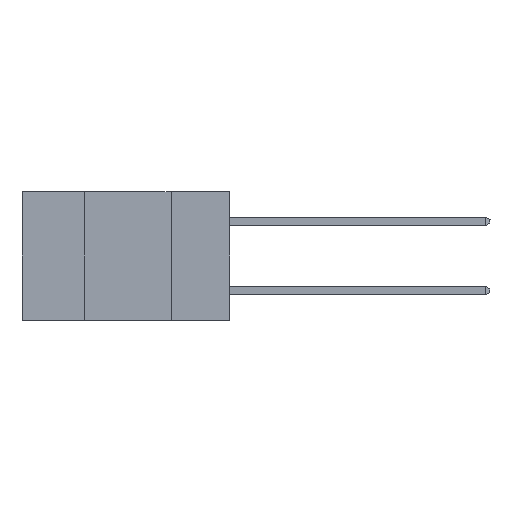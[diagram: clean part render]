
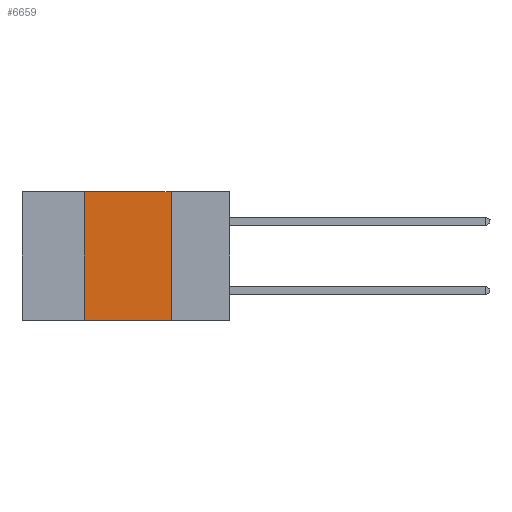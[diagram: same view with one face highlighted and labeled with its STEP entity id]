
A CAD part, left-side view. The second image highlights one B-rep face of the part: STEP entity #6659.
In plain terms, the highlighted planar face has unit normal (-1, 0, 0).
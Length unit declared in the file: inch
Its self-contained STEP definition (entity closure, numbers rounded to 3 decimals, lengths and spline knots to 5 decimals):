
#27 = DIRECTION ( 'NONE',  ( 0., 0., -1. ) ) ;
#76 = ORIENTED_EDGE ( 'NONE', *, *, #216, .T. ) ;
#216 = EDGE_CURVE ( 'NONE', #8223, #8405, #10692, .T. ) ;
#266 = CARTESIAN_POINT ( 'NONE',  ( 0., 0.17, 0. ) ) ;
#693 = EDGE_CURVE ( 'NONE', #8223, #9026, #9297, .T. ) ;
#1238 = DIRECTION ( 'NONE',  ( 1., 0., 0. ) ) ;
#1848 = VECTOR ( 'NONE', #7235, 39.37008 ) ;
#2009 = PLANE ( 'NONE',  #9515 ) ;
#2565 = EDGE_CURVE ( 'NONE', #7251, #8405, #10764, .T. ) ;
#2962 = DIRECTION ( 'NONE',  ( 0., -1., 0. ) ) ;
#3713 = VECTOR ( 'NONE', #4047, 39.37008 ) ;
#4047 = DIRECTION ( 'NONE',  ( 0., -1., 0. ) ) ;
#5865 = CARTESIAN_POINT ( 'NONE',  ( 0., 0.6, 0. ) ) ;
#6057 = FACE_OUTER_BOUND ( 'NONE', #9558, .T. ) ;
#6088 = ORIENTED_EDGE ( 'NONE', *, *, #9308, .F. ) ;
#6227 = CARTESIAN_POINT ( 'NONE',  ( 0., 0.42, -0.37 ) ) ;
#6659 = ADVANCED_FACE ( 'NONE', ( #6057 ), #2009, .F. ) ;
#7235 = DIRECTION ( 'NONE',  ( 0., 0., 1. ) ) ;
#7251 = VERTEX_POINT ( 'NONE', #266 ) ;
#7565 = CARTESIAN_POINT ( 'NONE',  ( 0., 0.42, -0.37 ) ) ;
#7998 = CARTESIAN_POINT ( 'NONE',  ( 0., 0.17, -0.37 ) ) ;
#8223 = VERTEX_POINT ( 'NONE', #7565 ) ;
#8405 = VERTEX_POINT ( 'NONE', #7998 ) ;
#8613 = VECTOR ( 'NONE', #2962, 39.37008 ) ;
#8817 = LINE ( 'NONE', #11612, #3713 ) ;
#8828 = CARTESIAN_POINT ( 'NONE',  ( 0., 0.17, -0.37 ) ) ;
#9026 = VERTEX_POINT ( 'NONE', #11838 ) ;
#9297 = LINE ( 'NONE', #6227, #1848 ) ;
#9308 = EDGE_CURVE ( 'NONE', #9026, #7251, #8817, .T. ) ;
#9362 = ORIENTED_EDGE ( 'NONE', *, *, #2565, .F. ) ;
#9515 = AXIS2_PLACEMENT_3D ( 'NONE', #5865, #1238, #27 ) ;
#9558 = EDGE_LOOP ( 'NONE', ( #9362, #6088, #11256, #76 ) ) ;
#9844 = VECTOR ( 'NONE', #11621, 39.37008 ) ;
#10692 = LINE ( 'NONE', #11680, #8613 ) ;
#10764 = LINE ( 'NONE', #8828, #9844 ) ;
#11256 = ORIENTED_EDGE ( 'NONE', *, *, #693, .F. ) ;
#11612 = CARTESIAN_POINT ( 'NONE',  ( 0., 0.6, 0. ) ) ;
#11621 = DIRECTION ( 'NONE',  ( 0., 0., -1. ) ) ;
#11680 = CARTESIAN_POINT ( 'NONE',  ( 0., 0.6, -0.37 ) ) ;
#11838 = CARTESIAN_POINT ( 'NONE',  ( 0., 0.42, 0. ) ) ;
